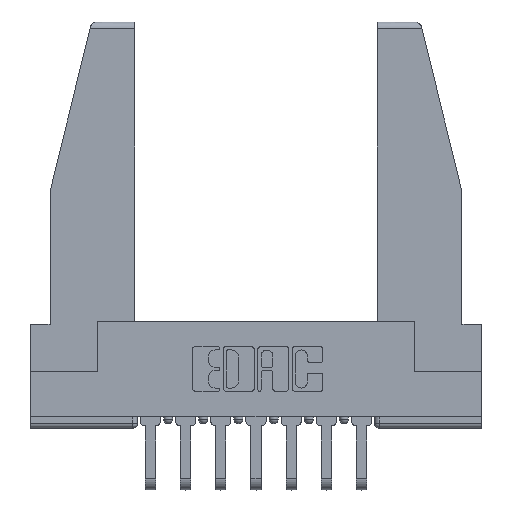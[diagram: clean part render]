
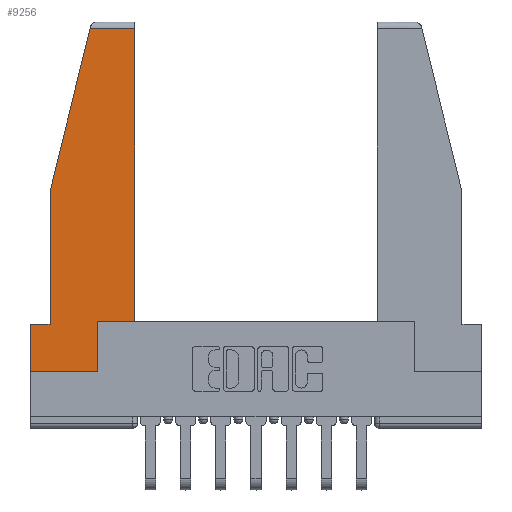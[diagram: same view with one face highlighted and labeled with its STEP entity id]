
A CAD part, top view. The second image highlights one B-rep face of the part: STEP entity #9256.
In plain terms, the highlighted planar face has unit normal (0, 0, 1).
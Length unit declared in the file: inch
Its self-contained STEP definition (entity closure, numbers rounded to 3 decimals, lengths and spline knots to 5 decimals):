
#518 = DIRECTION ( 'NONE',  ( 0., 0., 1. ) ) ;
#545 = EDGE_CURVE ( 'NONE', #3474, #7529, #7137, .T. ) ;
#874 = VECTOR ( 'NONE', #4558, 39.37008 ) ;
#1257 = EDGE_CURVE ( 'NONE', #6458, #12664, #1853, .T. ) ;
#1266 = ORIENTED_EDGE ( 'NONE', *, *, #2564, .T. ) ;
#1272 = ORIENTED_EDGE ( 'NONE', *, *, #1257, .T. ) ;
#1480 = CARTESIAN_POINT ( 'NONE',  ( 0.086, 0.8, 0. ) ) ;
#1853 = LINE ( 'NONE', #8797, #3061 ) ;
#2007 = CARTESIAN_POINT ( 'NONE',  ( 0.297, 0., 0. ) ) ;
#2326 = FACE_OUTER_BOUND ( 'NONE', #4465, .T. ) ;
#2433 = DIRECTION ( 'NONE',  ( 0., -1., 0. ) ) ;
#2564 = EDGE_CURVE ( 'NONE', #14445, #13498, #14072, .T. ) ;
#2645 = CARTESIAN_POINT ( 'NONE',  ( 0., 0.21, 0. ) ) ;
#2739 = LINE ( 'NONE', #9058, #4211 ) ;
#3061 = VECTOR ( 'NONE', #3308, 39.37008 ) ;
#3283 = CARTESIAN_POINT ( 'NONE',  ( 0., 1.52, 0. ) ) ;
#3308 = DIRECTION ( 'NONE',  ( -0.239, -0.971, 0. ) ) ;
#3348 = AXIS2_PLACEMENT_3D ( 'NONE', #11775, #518, #5096 ) ;
#3474 = VERTEX_POINT ( 'NONE', #6629 ) ;
#3996 = DIRECTION ( 'NONE',  ( 0., 1., 0. ) ) ;
#4077 = ORIENTED_EDGE ( 'NONE', *, *, #545, .T. ) ;
#4175 = VECTOR ( 'NONE', #3996, 39.37008 ) ;
#4211 = VECTOR ( 'NONE', #11314, 39.37008 ) ;
#4294 = CARTESIAN_POINT ( 'NONE',  ( 0.297, 0.223, 0. ) ) ;
#4369 = VERTEX_POINT ( 'NONE', #6740 ) ;
#4465 = EDGE_LOOP ( 'NONE', ( #11134, #9931, #1272, #11187, #1266, #4846, #4746, #4077, #7909 ) ) ;
#4492 = DIRECTION ( 'NONE',  ( 1., 0., 0. ) ) ;
#4558 = DIRECTION ( 'NONE',  ( -1., 0., 0. ) ) ;
#4746 = ORIENTED_EDGE ( 'NONE', *, *, #13866, .T. ) ;
#4846 = ORIENTED_EDGE ( 'NONE', *, *, #12498, .T. ) ;
#5096 = DIRECTION ( 'NONE',  ( 1., 0., 0. ) ) ;
#5550 = CARTESIAN_POINT ( 'NONE',  ( 0., 0., 0. ) ) ;
#5856 = CARTESIAN_POINT ( 'NONE',  ( 0., 0.21, 0. ) ) ;
#6052 = EDGE_CURVE ( 'NONE', #7529, #4369, #7344, .T. ) ;
#6458 = VERTEX_POINT ( 'NONE', #8900 ) ;
#6629 = CARTESIAN_POINT ( 'NONE',  ( 0.297, 0., 0. ) ) ;
#6740 = CARTESIAN_POINT ( 'NONE',  ( 0.461, 0.223, 0. ) ) ;
#6957 = EDGE_CURVE ( 'NONE', #4369, #10667, #8009, .T. ) ;
#7137 = LINE ( 'NONE', #2007, #9392 ) ;
#7344 = LINE ( 'NONE', #12253, #9603 ) ;
#7529 = VERTEX_POINT ( 'NONE', #4294 ) ;
#7714 = VERTEX_POINT ( 'NONE', #5550 ) ;
#7909 = ORIENTED_EDGE ( 'NONE', *, *, #6052, .T. ) ;
#8009 = LINE ( 'NONE', #9663, #4175 ) ;
#8018 = LINE ( 'NONE', #3283, #874 ) ;
#8162 = VECTOR ( 'NONE', #11901, 39.37008 ) ;
#8741 = VECTOR ( 'NONE', #2433, 39.37008 ) ;
#8797 = CARTESIAN_POINT ( 'NONE',  ( 0.271, 1.55, 0. ) ) ;
#8900 = CARTESIAN_POINT ( 'NONE',  ( 0.2636, 1.52, 0. ) ) ;
#9058 = CARTESIAN_POINT ( 'NONE',  ( 0., 0.21, 0. ) ) ;
#9256 = ADVANCED_FACE ( 'NONE', ( #2326 ), #10683, .T. ) ;
#9392 = VECTOR ( 'NONE', #12074, 39.37008 ) ;
#9451 = DIRECTION ( 'NONE',  ( -1., 0., 0. ) ) ;
#9603 = VECTOR ( 'NONE', #4492, 39.37008 ) ;
#9663 = CARTESIAN_POINT ( 'NONE',  ( 0.461, 0.223, 0. ) ) ;
#9931 = ORIENTED_EDGE ( 'NONE', *, *, #12349, .T. ) ;
#10667 = VERTEX_POINT ( 'NONE', #12314 ) ;
#10683 = PLANE ( 'NONE',  #3348 ) ;
#10809 = CARTESIAN_POINT ( 'NONE',  ( 0., 0., 0. ) ) ;
#11099 = VECTOR ( 'NONE', #9451, 39.37008 ) ;
#11134 = ORIENTED_EDGE ( 'NONE', *, *, #6957, .T. ) ;
#11187 = ORIENTED_EDGE ( 'NONE', *, *, #11197, .T. ) ;
#11197 = EDGE_CURVE ( 'NONE', #12664, #14445, #14180, .T. ) ;
#11314 = DIRECTION ( 'NONE',  ( 0., -1., 0. ) ) ;
#11318 = LINE ( 'NONE', #10809, #8162 ) ;
#11775 = CARTESIAN_POINT ( 'NONE',  ( 0., 0., 0. ) ) ;
#11901 = DIRECTION ( 'NONE',  ( 1., 0., 0. ) ) ;
#12032 = CARTESIAN_POINT ( 'NONE',  ( 0.086, 0.21, 0. ) ) ;
#12074 = DIRECTION ( 'NONE',  ( 0., 1., 0. ) ) ;
#12165 = CARTESIAN_POINT ( 'NONE',  ( 0.086, 0.8, 0. ) ) ;
#12253 = CARTESIAN_POINT ( 'NONE',  ( 0.297, 0.223, 0. ) ) ;
#12314 = CARTESIAN_POINT ( 'NONE',  ( 0.461, 1.52, 0. ) ) ;
#12349 = EDGE_CURVE ( 'NONE', #10667, #6458, #8018, .T. ) ;
#12498 = EDGE_CURVE ( 'NONE', #13498, #7714, #2739, .T. ) ;
#12664 = VERTEX_POINT ( 'NONE', #1480 ) ;
#13498 = VERTEX_POINT ( 'NONE', #5856 ) ;
#13866 = EDGE_CURVE ( 'NONE', #7714, #3474, #11318, .T. ) ;
#14072 = LINE ( 'NONE', #2645, #11099 ) ;
#14180 = LINE ( 'NONE', #12165, #8741 ) ;
#14445 = VERTEX_POINT ( 'NONE', #12032 ) ;
